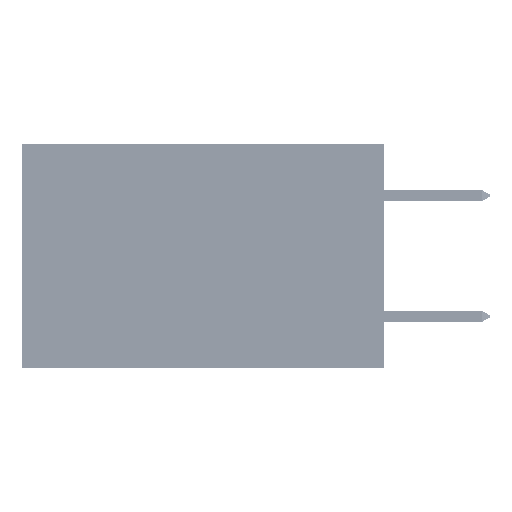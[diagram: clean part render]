
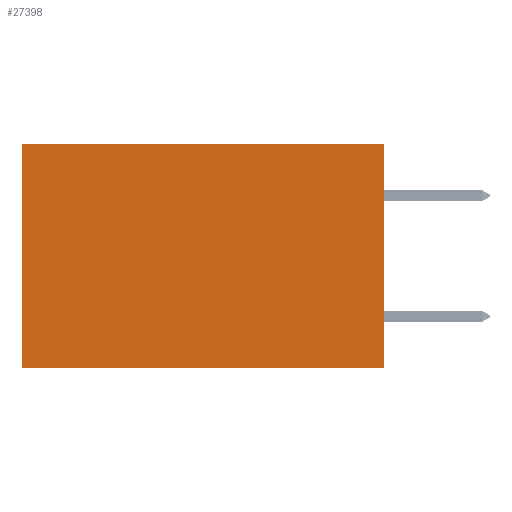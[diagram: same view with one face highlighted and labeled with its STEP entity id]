
A CAD part, left-side view. The second image highlights one B-rep face of the part: STEP entity #27398.
In plain terms, the highlighted planar face has unit normal (-1, 0, 0).
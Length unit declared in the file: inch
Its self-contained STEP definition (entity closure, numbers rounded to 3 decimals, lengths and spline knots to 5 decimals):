
#290 = ORIENTED_EDGE ( 'NONE', *, *, #15996, .T. ) ;
#1191 = VERTEX_POINT ( 'NONE', #48126 ) ;
#4217 = EDGE_CURVE ( 'NONE', #1191, #47558, #37546, .T. ) ;
#5548 = PLANE ( 'NONE',  #46127 ) ;
#7678 = CARTESIAN_POINT ( 'NONE',  ( 0.2875, 0., -0.37 ) ) ;
#8986 = DIRECTION ( 'NONE',  ( 0., 0., -1. ) ) ;
#11298 = FACE_OUTER_BOUND ( 'NONE', #30924, .T. ) ;
#13435 = CARTESIAN_POINT ( 'NONE',  ( 0.2875, 0.6, -0.37 ) ) ;
#13600 = EDGE_CURVE ( 'NONE', #21096, #27424, #17040, .T. ) ;
#15996 = EDGE_CURVE ( 'NONE', #47558, #27424, #28285, .T. ) ;
#17040 = LINE ( 'NONE', #7678, #46452 ) ;
#19863 = CARTESIAN_POINT ( 'NONE',  ( 0.2875, 0., 0. ) ) ;
#21096 = VERTEX_POINT ( 'NONE', #46394 ) ;
#27370 = ORIENTED_EDGE ( 'NONE', *, *, #13600, .F. ) ;
#27398 = ADVANCED_FACE ( 'NONE', ( #11298 ), #5548, .F. ) ;
#27424 = VERTEX_POINT ( 'NONE', #13435 ) ;
#27777 = EDGE_CURVE ( 'NONE', #1191, #21096, #49151, .T. ) ;
#28285 = LINE ( 'NONE', #39361, #43886 ) ;
#30924 = EDGE_LOOP ( 'NONE', ( #290, #27370, #44787, #41087 ) ) ;
#34705 = DIRECTION ( 'NONE',  ( 0., 1., 0. ) ) ;
#36076 = CARTESIAN_POINT ( 'NONE',  ( 0.2875, 0., 0. ) ) ;
#37546 = LINE ( 'NONE', #41807, #43523 ) ;
#38711 = CARTESIAN_POINT ( 'NONE',  ( 0.2875, 0.6, 0. ) ) ;
#38877 = VECTOR ( 'NONE', #46710, 39.37008 ) ;
#39361 = CARTESIAN_POINT ( 'NONE',  ( 0.2875, 0.6, 0. ) ) ;
#40116 = DIRECTION ( 'NONE',  ( 0., 0., -1. ) ) ;
#41087 = ORIENTED_EDGE ( 'NONE', *, *, #4217, .T. ) ;
#41807 = CARTESIAN_POINT ( 'NONE',  ( 0.2875, 0., 0. ) ) ;
#43523 = VECTOR ( 'NONE', #45967, 39.37008 ) ;
#43886 = VECTOR ( 'NONE', #8986, 39.37008 ) ;
#44787 = ORIENTED_EDGE ( 'NONE', *, *, #27777, .F. ) ;
#45967 = DIRECTION ( 'NONE',  ( 0., 1., 0. ) ) ;
#46127 = AXIS2_PLACEMENT_3D ( 'NONE', #36076, #48027, #40116 ) ;
#46394 = CARTESIAN_POINT ( 'NONE',  ( 0.2875, 0., -0.37 ) ) ;
#46452 = VECTOR ( 'NONE', #34705, 39.37008 ) ;
#46710 = DIRECTION ( 'NONE',  ( 0., 0., -1. ) ) ;
#47558 = VERTEX_POINT ( 'NONE', #38711 ) ;
#48027 = DIRECTION ( 'NONE',  ( 1., 0., 0. ) ) ;
#48126 = CARTESIAN_POINT ( 'NONE',  ( 0.2875, 0., 0. ) ) ;
#49151 = LINE ( 'NONE', #19863, #38877 ) ;
